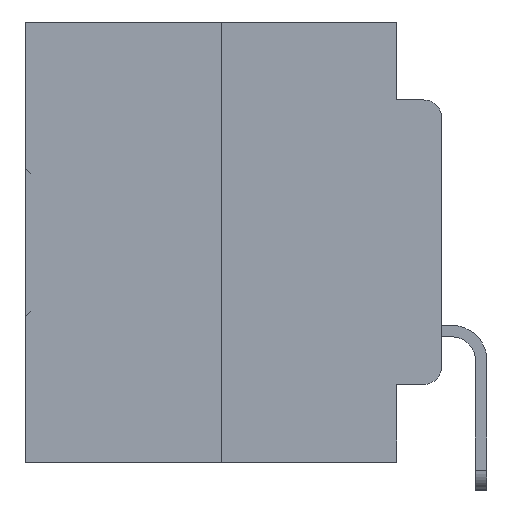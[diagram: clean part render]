
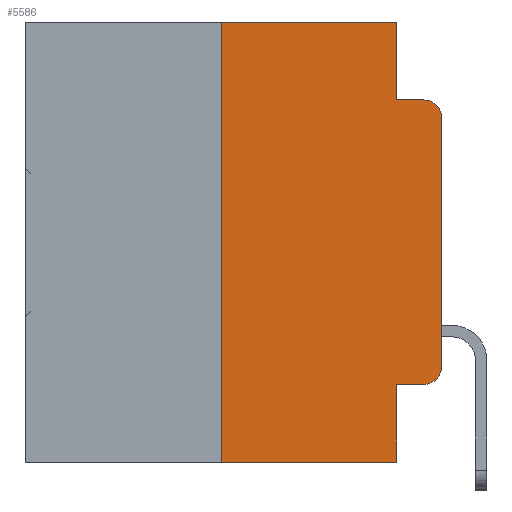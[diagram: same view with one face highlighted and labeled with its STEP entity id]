
A CAD part, left-side view. The second image highlights one B-rep face of the part: STEP entity #5586.
In plain terms, the highlighted planar face has unit normal (-1, 0, 0).
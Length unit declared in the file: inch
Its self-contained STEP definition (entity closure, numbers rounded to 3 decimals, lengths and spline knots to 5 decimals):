
#201 = VERTEX_POINT ( 'NONE', #23758 ) ;
#491 = AXIS2_PLACEMENT_3D ( 'NONE', #31476, #16948, #1302 ) ;
#523 = EDGE_CURVE ( 'NONE', #20418, #15595, #6003, .T. ) ;
#710 = ORIENTED_EDGE ( 'NONE', *, *, #29998, .F. ) ;
#1123 = DIRECTION ( 'NONE',  ( 0., -1., 0. ) ) ;
#1136 = ORIENTED_EDGE ( 'NONE', *, *, #7700, .F. ) ;
#1302 = DIRECTION ( 'NONE',  ( 0., 0., -1. ) ) ;
#1587 = ORIENTED_EDGE ( 'NONE', *, *, #23599, .T. ) ;
#1721 = VECTOR ( 'NONE', #8067, 39.37008 ) ;
#2204 = CARTESIAN_POINT ( 'NONE',  ( 0., 0.051, -0.0885 ) ) ;
#2227 = VECTOR ( 'NONE', #14080, 39.37008 ) ;
#4107 = EDGE_CURVE ( 'NONE', #10987, #20418, #14336, .T. ) ;
#5586 = ADVANCED_FACE ( 'NONE', ( #25388 ), #29020, .F. ) ;
#6003 = LINE ( 'NONE', #26762, #31718 ) ;
#6767 = AXIS2_PLACEMENT_3D ( 'NONE', #28666, #14003, #31079 ) ;
#6769 = DIRECTION ( 'NONE',  ( 0., 0., 1. ) ) ;
#7392 = VECTOR ( 'NONE', #27311, 39.37008 ) ;
#7493 = CARTESIAN_POINT ( 'NONE',  ( 0., 0.051, -0.5 ) ) ;
#7700 = EDGE_CURVE ( 'NONE', #15595, #10801, #16772, .T. ) ;
#8067 = DIRECTION ( 'NONE',  ( 0., 0., -1. ) ) ;
#8976 = DIRECTION ( 'NONE',  ( 0., -1., 0. ) ) ;
#9191 = CARTESIAN_POINT ( 'NONE',  ( 0., 0.473, 0. ) ) ;
#9879 = ORIENTED_EDGE ( 'NONE', *, *, #4107, .F. ) ;
#9937 = VECTOR ( 'NONE', #6769, 39.37008 ) ;
#10058 = CARTESIAN_POINT ( 'NONE',  ( 0., 0.25, -0.5 ) ) ;
#10208 = CIRCLE ( 'NONE', #6767, 0.02 ) ;
#10801 = VERTEX_POINT ( 'NONE', #26343 ) ;
#10987 = VERTEX_POINT ( 'NONE', #31855 ) ;
#12075 = VERTEX_POINT ( 'NONE', #24765 ) ;
#12679 = ORIENTED_EDGE ( 'NONE', *, *, #14685, .T. ) ;
#13284 = CARTESIAN_POINT ( 'NONE',  ( 0., 0.051, 0. ) ) ;
#13728 = CARTESIAN_POINT ( 'NONE',  ( 0., 0.051, 0. ) ) ;
#14003 = DIRECTION ( 'NONE',  ( -1., 0., 0. ) ) ;
#14080 = DIRECTION ( 'NONE',  ( 0., -1., 0. ) ) ;
#14336 = LINE ( 'NONE', #32106, #7392 ) ;
#14390 = DIRECTION ( 'NONE',  ( 1., 0., 0. ) ) ;
#14685 = EDGE_CURVE ( 'NONE', #27159, #10801, #30392, .T. ) ;
#15069 = AXIS2_PLACEMENT_3D ( 'NONE', #9191, #14390, #31428 ) ;
#15337 = LINE ( 'NONE', #16373, #21966 ) ;
#15595 = VERTEX_POINT ( 'NONE', #2204 ) ;
#15652 = LINE ( 'NONE', #13284, #1721 ) ;
#15779 = EDGE_LOOP ( 'NONE', ( #18662, #12679, #1136, #28868, #9879, #24780, #31851, #710, #21394, #1587 ) ) ;
#15962 = EDGE_CURVE ( 'NONE', #19555, #29783, #16613, .T. ) ;
#16373 = CARTESIAN_POINT ( 'NONE',  ( 0., 0., 0. ) ) ;
#16613 = LINE ( 'NONE', #16792, #17388 ) ;
#16772 = LINE ( 'NONE', #24054, #17562 ) ;
#16792 = CARTESIAN_POINT ( 'NONE',  ( 0., 0.473, -0.5 ) ) ;
#16920 = LINE ( 'NONE', #21620, #2227 ) ;
#16948 = DIRECTION ( 'NONE',  ( -1., 0., 0. ) ) ;
#17037 = CARTESIAN_POINT ( 'NONE',  ( 0., 0.25, 0. ) ) ;
#17388 = VECTOR ( 'NONE', #1123, 39.37008 ) ;
#17544 = LINE ( 'NONE', #17037, #9937 ) ;
#17562 = VECTOR ( 'NONE', #8976, 39.37008 ) ;
#18049 = EDGE_CURVE ( 'NONE', #201, #27159, #15337, .T. ) ;
#18662 = ORIENTED_EDGE ( 'NONE', *, *, #18049, .T. ) ;
#18905 = DIRECTION ( 'NONE',  ( 0., 0., 1. ) ) ;
#19555 = VERTEX_POINT ( 'NONE', #10058 ) ;
#20418 = VERTEX_POINT ( 'NONE', #13728 ) ;
#21394 = ORIENTED_EDGE ( 'NONE', *, *, #25197, .T. ) ;
#21620 = CARTESIAN_POINT ( 'NONE',  ( 0., 0.051, -0.4115 ) ) ;
#21966 = VECTOR ( 'NONE', #18905, 39.37008 ) ;
#23052 = VERTEX_POINT ( 'NONE', #27125 ) ;
#23278 = CARTESIAN_POINT ( 'NONE',  ( 0., 0., -0.1085 ) ) ;
#23599 = EDGE_CURVE ( 'NONE', #23052, #201, #10208, .T. ) ;
#23758 = CARTESIAN_POINT ( 'NONE',  ( 0., 0., -0.3915 ) ) ;
#24054 = CARTESIAN_POINT ( 'NONE',  ( 0., 0.051, -0.0885 ) ) ;
#24765 = CARTESIAN_POINT ( 'NONE',  ( 0., 0.051, -0.4115 ) ) ;
#24780 = ORIENTED_EDGE ( 'NONE', *, *, #31604, .F. ) ;
#25197 = EDGE_CURVE ( 'NONE', #12075, #23052, #16920, .T. ) ;
#25388 = FACE_OUTER_BOUND ( 'NONE', #15779, .T. ) ;
#26343 = CARTESIAN_POINT ( 'NONE',  ( 0., 0.02, -0.0885 ) ) ;
#26728 = DIRECTION ( 'NONE',  ( 0., 0., -1. ) ) ;
#26762 = CARTESIAN_POINT ( 'NONE',  ( 0., 0.051, 0. ) ) ;
#27125 = CARTESIAN_POINT ( 'NONE',  ( 0., 0.02, -0.4115 ) ) ;
#27159 = VERTEX_POINT ( 'NONE', #23278 ) ;
#27311 = DIRECTION ( 'NONE',  ( 0., -1., 0. ) ) ;
#28666 = CARTESIAN_POINT ( 'NONE',  ( 0., 0.02, -0.3915 ) ) ;
#28868 = ORIENTED_EDGE ( 'NONE', *, *, #523, .F. ) ;
#29020 = PLANE ( 'NONE',  #15069 ) ;
#29783 = VERTEX_POINT ( 'NONE', #7493 ) ;
#29998 = EDGE_CURVE ( 'NONE', #12075, #29783, #15652, .T. ) ;
#30392 = CIRCLE ( 'NONE', #491, 0.02 ) ;
#31079 = DIRECTION ( 'NONE',  ( 0., 0., -1. ) ) ;
#31428 = DIRECTION ( 'NONE',  ( 0., 0., -1. ) ) ;
#31476 = CARTESIAN_POINT ( 'NONE',  ( 0., 0.02, -0.1085 ) ) ;
#31604 = EDGE_CURVE ( 'NONE', #19555, #10987, #17544, .T. ) ;
#31718 = VECTOR ( 'NONE', #26728, 39.37008 ) ;
#31851 = ORIENTED_EDGE ( 'NONE', *, *, #15962, .T. ) ;
#31855 = CARTESIAN_POINT ( 'NONE',  ( 0., 0.25, 0. ) ) ;
#32106 = CARTESIAN_POINT ( 'NONE',  ( 0., 0.473, 0. ) ) ;
